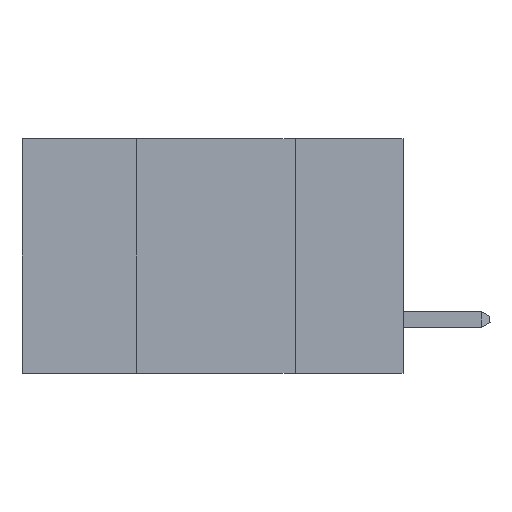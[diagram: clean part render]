
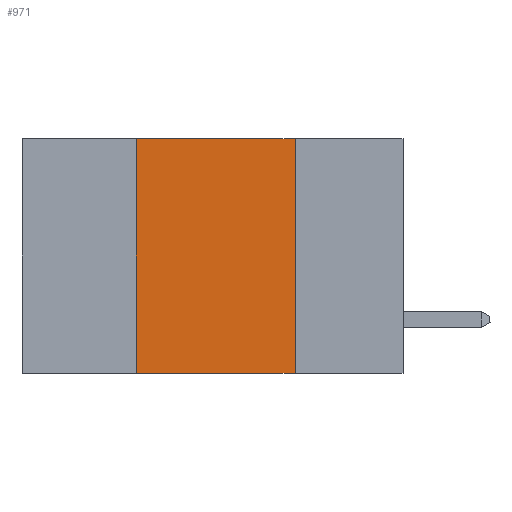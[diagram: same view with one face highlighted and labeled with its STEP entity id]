
A CAD part, left-side view. The second image highlights one B-rep face of the part: STEP entity #971.
In plain terms, the highlighted planar face has unit normal (-1, 0, 0).
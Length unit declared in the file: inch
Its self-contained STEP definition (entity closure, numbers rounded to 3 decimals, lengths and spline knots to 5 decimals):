
#705 = CARTESIAN_POINT ( 'NONE',  ( 0., 0.17, 0. ) ) ;
#971 = ADVANCED_FACE ( 'NONE', ( #11571 ), #11852, .F. ) ;
#1340 = CARTESIAN_POINT ( 'NONE',  ( 0., 0.6, 0. ) ) ;
#1405 = CARTESIAN_POINT ( 'NONE',  ( 0., 0.6, -0.37 ) ) ;
#1416 = DIRECTION ( 'NONE',  ( 0., 0., 1. ) ) ;
#1671 = VERTEX_POINT ( 'NONE', #4111 ) ;
#1959 = VERTEX_POINT ( 'NONE', #2568 ) ;
#2568 = CARTESIAN_POINT ( 'NONE',  ( 0., 0.42, 0. ) ) ;
#2722 = EDGE_LOOP ( 'NONE', ( #4682, #4775, #4246, #2745 ) ) ;
#2745 = ORIENTED_EDGE ( 'NONE', *, *, #3402, .T. ) ;
#2810 = EDGE_CURVE ( 'NONE', #5597, #1671, #4620, .T. ) ;
#3402 = EDGE_CURVE ( 'NONE', #10412, #1671, #4743, .T. ) ;
#3875 = DIRECTION ( 'NONE',  ( 0., -1., 0. ) ) ;
#4111 = CARTESIAN_POINT ( 'NONE',  ( 0., 0.17, -0.37 ) ) ;
#4246 = ORIENTED_EDGE ( 'NONE', *, *, #9469, .F. ) ;
#4465 = VECTOR ( 'NONE', #12051, 39.37008 ) ;
#4620 = LINE ( 'NONE', #9080, #4910 ) ;
#4682 = ORIENTED_EDGE ( 'NONE', *, *, #2810, .F. ) ;
#4743 = LINE ( 'NONE', #1405, #4465 ) ;
#4775 = ORIENTED_EDGE ( 'NONE', *, *, #6338, .F. ) ;
#4910 = VECTOR ( 'NONE', #7262, 39.37008 ) ;
#4966 = DIRECTION ( 'NONE',  ( 1., 0., 0. ) ) ;
#5597 = VERTEX_POINT ( 'NONE', #705 ) ;
#6338 = EDGE_CURVE ( 'NONE', #1959, #5597, #9082, .T. ) ;
#6436 = LINE ( 'NONE', #8251, #10377 ) ;
#6667 = CARTESIAN_POINT ( 'NONE',  ( 0., 0.6, 0. ) ) ;
#7262 = DIRECTION ( 'NONE',  ( 0., 0., -1. ) ) ;
#8251 = CARTESIAN_POINT ( 'NONE',  ( 0., 0.42, 0. ) ) ;
#9080 = CARTESIAN_POINT ( 'NONE',  ( 0., 0.17, 0. ) ) ;
#9082 = LINE ( 'NONE', #6667, #10447 ) ;
#9469 = EDGE_CURVE ( 'NONE', #10412, #1959, #6436, .T. ) ;
#10253 = AXIS2_PLACEMENT_3D ( 'NONE', #1340, #4966, #11932 ) ;
#10377 = VECTOR ( 'NONE', #1416, 39.37008 ) ;
#10412 = VERTEX_POINT ( 'NONE', #12237 ) ;
#10447 = VECTOR ( 'NONE', #3875, 39.37008 ) ;
#11571 = FACE_OUTER_BOUND ( 'NONE', #2722, .T. ) ;
#11852 = PLANE ( 'NONE',  #10253 ) ;
#11932 = DIRECTION ( 'NONE',  ( 0., 0., -1. ) ) ;
#12051 = DIRECTION ( 'NONE',  ( 0., -1., 0. ) ) ;
#12237 = CARTESIAN_POINT ( 'NONE',  ( 0., 0.42, -0.37 ) ) ;
